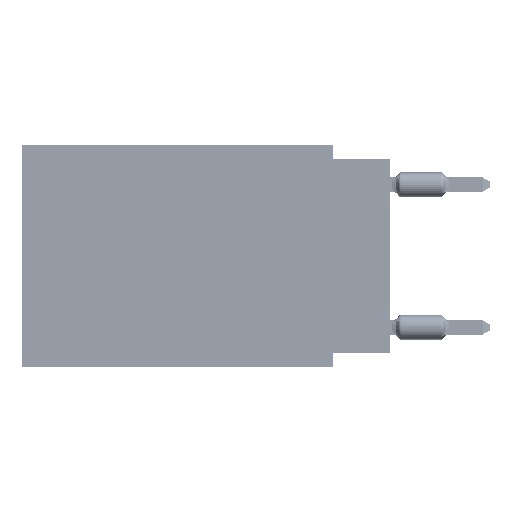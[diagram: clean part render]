
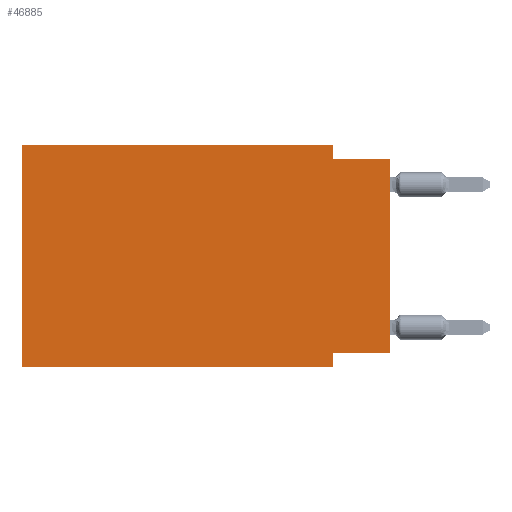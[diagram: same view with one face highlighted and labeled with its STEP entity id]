
A CAD part, left-side view. The second image highlights one B-rep face of the part: STEP entity #46885.
In plain terms, the highlighted planar face has unit normal (-1, 0, 0).
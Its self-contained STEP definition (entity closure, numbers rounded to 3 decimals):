
#3386 = CARTESIAN_POINT ( 'NONE',  ( 0., 16.383, -9.906 ) ) ;
#4111 = PLANE ( 'NONE',  #45825 ) ;
#4463 = CARTESIAN_POINT ( 'NONE',  ( 0., 16.383, 0. ) ) ;
#4543 = VERTEX_POINT ( 'NONE', #82389 ) ;
#5419 = VECTOR ( 'NONE', #76892, 1000. ) ;
#6489 = EDGE_LOOP ( 'NONE', ( #82310, #31306, #46755, #15168, #11494, #61087, #87447, #87240 ) ) ;
#7853 = CARTESIAN_POINT ( 'NONE',  ( 0., 16.383, 0. ) ) ;
#10020 = LINE ( 'NONE', #3386, #64999 ) ;
#10597 = CARTESIAN_POINT ( 'NONE',  ( 0., 2.54, -9.906 ) ) ;
#11267 = VECTOR ( 'NONE', #25985, 1000. ) ;
#11494 = ORIENTED_EDGE ( 'NONE', *, *, #33449, .F. ) ;
#12370 = FACE_OUTER_BOUND ( 'NONE', #6489, .T. ) ;
#13680 = DIRECTION ( 'NONE',  ( 0., -1., 0. ) ) ;
#15168 = ORIENTED_EDGE ( 'NONE', *, *, #32963, .F. ) ;
#15420 = VECTOR ( 'NONE', #67110, 1000. ) ;
#15776 = EDGE_CURVE ( 'NONE', #49049, #80752, #66894, .T. ) ;
#15870 = EDGE_CURVE ( 'NONE', #36829, #80752, #10020, .T. ) ;
#16721 = LINE ( 'NONE', #42842, #5419 ) ;
#18159 = LINE ( 'NONE', #4463, #60557 ) ;
#21189 = CARTESIAN_POINT ( 'NONE',  ( 0., 0., -0.635 ) ) ;
#25643 = DIRECTION ( 'NONE',  ( 1., 0., 0. ) ) ;
#25953 = EDGE_CURVE ( 'NONE', #4543, #83193, #27132, .T. ) ;
#25985 = DIRECTION ( 'NONE',  ( 0., 0., -1. ) ) ;
#26249 = DIRECTION ( 'NONE',  ( 0., 0., 1. ) ) ;
#27132 = LINE ( 'NONE', #81101, #76899 ) ;
#29869 = VERTEX_POINT ( 'NONE', #85071 ) ;
#31087 = CARTESIAN_POINT ( 'NONE',  ( 0., 16.383, 0. ) ) ;
#31241 = DIRECTION ( 'NONE',  ( 0., -1., 0. ) ) ;
#31306 = ORIENTED_EDGE ( 'NONE', *, *, #71472, .F. ) ;
#32189 = EDGE_CURVE ( 'NONE', #66333, #29869, #72870, .T. ) ;
#32963 = EDGE_CURVE ( 'NONE', #33549, #66333, #18159, .T. ) ;
#33449 = EDGE_CURVE ( 'NONE', #36829, #33549, #39712, .T. ) ;
#33549 = VERTEX_POINT ( 'NONE', #7853 ) ;
#36829 = VERTEX_POINT ( 'NONE', #80644 ) ;
#37439 = CARTESIAN_POINT ( 'NONE',  ( 0., 2.54, -9.906 ) ) ;
#39712 = LINE ( 'NONE', #66657, #15420 ) ;
#42842 = CARTESIAN_POINT ( 'NONE',  ( 0., 0., -9.271 ) ) ;
#43502 = DIRECTION ( 'NONE',  ( 0., 0., -1. ) ) ;
#43837 = CARTESIAN_POINT ( 'NONE',  ( 0., 0., -0.635 ) ) ;
#45151 = DIRECTION ( 'NONE',  ( 0., -1., 0. ) ) ;
#45825 = AXIS2_PLACEMENT_3D ( 'NONE', #31087, #25643, #43502 ) ;
#46755 = ORIENTED_EDGE ( 'NONE', *, *, #32189, .F. ) ;
#46885 = ADVANCED_FACE ( 'NONE', ( #12370 ), #4111, .F. ) ;
#49049 = VERTEX_POINT ( 'NONE', #78104 ) ;
#60557 = VECTOR ( 'NONE', #45151, 1000. ) ;
#61087 = ORIENTED_EDGE ( 'NONE', *, *, #15870, .T. ) ;
#64267 = CARTESIAN_POINT ( 'NONE',  ( 0., 2.54, 0. ) ) ;
#64999 = VECTOR ( 'NONE', #31241, 1000. ) ;
#66333 = VERTEX_POINT ( 'NONE', #64267 ) ;
#66657 = CARTESIAN_POINT ( 'NONE',  ( 0., 16.383, 0. ) ) ;
#66894 = LINE ( 'NONE', #37439, #74932 ) ;
#67110 = DIRECTION ( 'NONE',  ( 0., 0., 1. ) ) ;
#71472 = EDGE_CURVE ( 'NONE', #29869, #83193, #81788, .T. ) ;
#72870 = LINE ( 'NONE', #73288, #11267 ) ;
#73288 = CARTESIAN_POINT ( 'NONE',  ( 0., 2.54, 0. ) ) ;
#74722 = EDGE_CURVE ( 'NONE', #4543, #49049, #16721, .T. ) ;
#74932 = VECTOR ( 'NONE', #84775, 1000. ) ;
#76892 = DIRECTION ( 'NONE',  ( 0., 1., 0. ) ) ;
#76899 = VECTOR ( 'NONE', #26249, 1000. ) ;
#78104 = CARTESIAN_POINT ( 'NONE',  ( 0., 2.54, -9.271 ) ) ;
#80644 = CARTESIAN_POINT ( 'NONE',  ( 0., 16.383, -9.906 ) ) ;
#80752 = VERTEX_POINT ( 'NONE', #10597 ) ;
#81101 = CARTESIAN_POINT ( 'NONE',  ( 0., 0., 0. ) ) ;
#81788 = LINE ( 'NONE', #21189, #84375 ) ;
#82310 = ORIENTED_EDGE ( 'NONE', *, *, #25953, .T. ) ;
#82389 = CARTESIAN_POINT ( 'NONE',  ( 0., 0., -9.271 ) ) ;
#83193 = VERTEX_POINT ( 'NONE', #43837 ) ;
#84375 = VECTOR ( 'NONE', #13680, 1000. ) ;
#84775 = DIRECTION ( 'NONE',  ( 0., 0., -1. ) ) ;
#85071 = CARTESIAN_POINT ( 'NONE',  ( 0., 2.54, -0.635 ) ) ;
#87240 = ORIENTED_EDGE ( 'NONE', *, *, #74722, .F. ) ;
#87447 = ORIENTED_EDGE ( 'NONE', *, *, #15776, .F. ) ;
